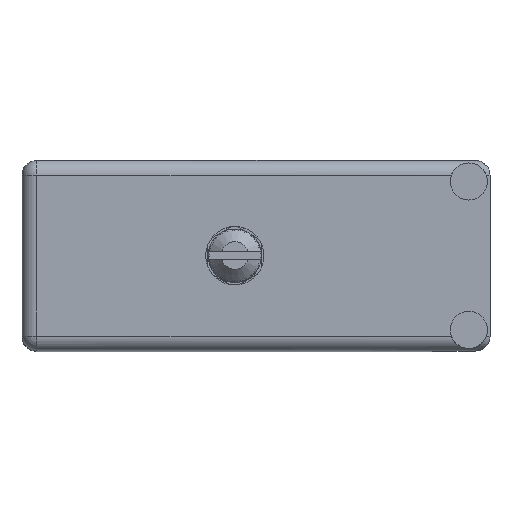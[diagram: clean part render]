
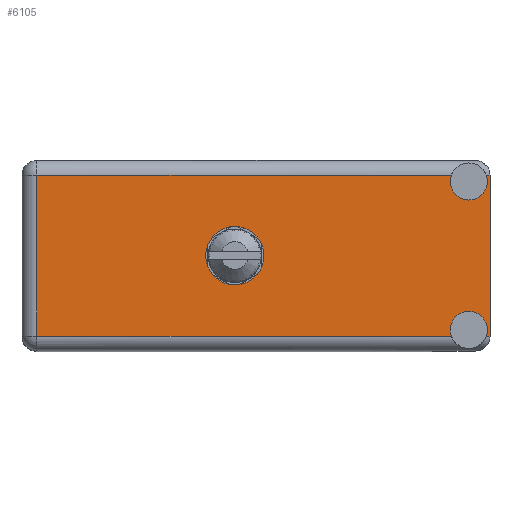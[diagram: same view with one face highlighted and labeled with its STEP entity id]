
A CAD part, top view. The second image highlights one B-rep face of the part: STEP entity #6105.
In plain terms, the highlighted face is planar.
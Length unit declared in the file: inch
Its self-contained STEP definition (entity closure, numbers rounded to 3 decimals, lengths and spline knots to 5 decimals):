
#167 = EDGE_CURVE ( 'NONE', #18167, #98111, #81407, .T. ) ;
#2049 = ORIENTED_EDGE ( 'NONE', *, *, #29045, .T. ) ;
#2720 = CIRCLE ( 'NONE', #59453, 0.0875 ) ;
#3264 = DIRECTION ( 'NONE',  ( 0., 0., 1. ) ) ;
#5481 = CARTESIAN_POINT ( 'NONE',  ( 2.108, 1.566, -0.0995 ) ) ;
#6029 = DIRECTION ( 'NONE',  ( 1., 0., 0. ) ) ;
#6105 = ADVANCED_FACE ( 'NONE', ( #53338, #6647 ), #45706, .T. ) ;
#6292 = VECTOR ( 'NONE', #83411, 39.37008 ) ;
#6294 = AXIS2_PLACEMENT_3D ( 'NONE', #74366, #57599, #89124 ) ;
#6647 = FACE_OUTER_BOUND ( 'NONE', #37424, .T. ) ;
#7308 = DIRECTION ( 'NONE',  ( 0., 0., 1. ) ) ;
#8499 = VERTEX_POINT ( 'NONE', #96741 ) ;
#9598 = ORIENTED_EDGE ( 'NONE', *, *, #73943, .T. ) ;
#11935 = ORIENTED_EDGE ( 'NONE', *, *, #15092, .F. ) ;
#12194 = VERTEX_POINT ( 'NONE', #40960 ) ;
#14160 = VECTOR ( 'NONE', #81929, 39.37008 ) ;
#14945 = ORIENTED_EDGE ( 'NONE', *, *, #33835, .F. ) ;
#15092 = EDGE_CURVE ( 'NONE', #77803, #8499, #61618, .T. ) ;
#16746 = CARTESIAN_POINT ( 'NONE',  ( 2.02562, 1.566, -0.07 ) ) ;
#18047 = EDGE_CURVE ( 'NONE', #32101, #18167, #29146, .T. ) ;
#18167 = VERTEX_POINT ( 'NONE', #63089 ) ;
#18726 = DIRECTION ( 'NONE',  ( 0., 1., 0. ) ) ;
#19003 = DIRECTION ( 'NONE',  ( 0., 1., 0. ) ) ;
#19771 = CARTESIAN_POINT ( 'NONE',  ( 2.108, 1.566, -0.0995 ) ) ;
#21005 = CARTESIAN_POINT ( 'NONE',  ( 1.004, 1.566, -0.312 ) ) ;
#23653 = AXIS2_PLACEMENT_3D ( 'NONE', #79051, #95802, #87690 ) ;
#26522 = VECTOR ( 'NONE', #88206, 39.37008 ) ;
#28844 = VERTEX_POINT ( 'NONE', #21005 ) ;
#28890 = CIRCLE ( 'NONE', #41594, 0.1375 ) ;
#29045 = EDGE_CURVE ( 'NONE', #98111, #50592, #42604, .T. ) ;
#29146 = LINE ( 'NONE', #60066, #6292 ) ;
#29497 = DIRECTION ( 'NONE',  ( 0., 0., 1. ) ) ;
#29644 = CARTESIAN_POINT ( 'NONE',  ( 0.07, 1.566, -0.07 ) ) ;
#32101 = VERTEX_POINT ( 'NONE', #44462 ) ;
#32908 = ORIENTED_EDGE ( 'NONE', *, *, #60147, .T. ) ;
#33835 = EDGE_CURVE ( 'NONE', #32101, #92286, #97107, .T. ) ;
#33897 = CARTESIAN_POINT ( 'NONE',  ( 0., 1.566, -0.829 ) ) ;
#36621 = VECTOR ( 'NONE', #6029, 39.37008 ) ;
#37424 = EDGE_LOOP ( 'NONE', ( #2049, #88988, #90297, #32908, #11935, #9598, #80236, #14945, #94966, #97171 ) ) ;
#37612 = DIRECTION ( 'NONE',  ( 0., 1., 0. ) ) ;
#40960 = CARTESIAN_POINT ( 'NONE',  ( 2.19038, 1.566, -0.829 ) ) ;
#41594 = AXIS2_PLACEMENT_3D ( 'NONE', #70141, #61550, #92561 ) ;
#41675 = AXIS2_PLACEMENT_3D ( 'NONE', #90568, #19003, #3264 ) ;
#42604 = LINE ( 'NONE', #90348, #84325 ) ;
#44462 = CARTESIAN_POINT ( 'NONE',  ( 2.02562, 1.566, -0.829 ) ) ;
#45706 = PLANE ( 'NONE',  #98157 ) ;
#46573 = EDGE_CURVE ( 'NONE', #28844, #48893, #83858, .T. ) ;
#48128 = EDGE_CURVE ( 'NONE', #48893, #28844, #28890, .T. ) ;
#48893 = VERTEX_POINT ( 'NONE', #71758 ) ;
#48980 = ORIENTED_EDGE ( 'NONE', *, *, #46573, .F. ) ;
#49653 = DIRECTION ( 'NONE',  ( 0., 0., 1. ) ) ;
#50592 = VERTEX_POINT ( 'NONE', #16746 ) ;
#51192 = DIRECTION ( 'NONE',  ( 0., 1., 0. ) ) ;
#52324 = CARTESIAN_POINT ( 'NONE',  ( 2.108, 1.566, -0.187 ) ) ;
#52597 = VERTEX_POINT ( 'NONE', #52324 ) ;
#53338 = FACE_BOUND ( 'NONE', #90382, .T. ) ;
#53491 = CARTESIAN_POINT ( 'NONE',  ( 2.208, 1.566, 0. ) ) ;
#57599 = DIRECTION ( 'NONE',  ( 0., 1., 0. ) ) ;
#58346 = DIRECTION ( 'NONE',  ( 1., 0., 0. ) ) ;
#59453 = AXIS2_PLACEMENT_3D ( 'NONE', #19771, #51192, #66448 ) ;
#60066 = CARTESIAN_POINT ( 'NONE',  ( 0., 1.566, -0.829 ) ) ;
#60147 = EDGE_CURVE ( 'NONE', #83844, #8499, #83677, .T. ) ;
#60887 = VECTOR ( 'NONE', #7308, 39.37008 ) ;
#61550 = DIRECTION ( 'NONE',  ( 0., 1., 0. ) ) ;
#61618 = LINE ( 'NONE', #53491, #60887 ) ;
#63089 = CARTESIAN_POINT ( 'NONE',  ( 0.07, 1.566, -0.829 ) ) ;
#64164 = EDGE_CURVE ( 'NONE', #52597, #50592, #96614, .T. ) ;
#64333 = LINE ( 'NONE', #33897, #26522 ) ;
#65685 = CARTESIAN_POINT ( 'NONE',  ( 0.07, 1.566, -0.899 ) ) ;
#65789 = AXIS2_PLACEMENT_3D ( 'NONE', #5481, #18726, #49653 ) ;
#66448 = DIRECTION ( 'NONE',  ( 0., 0., 1. ) ) ;
#69837 = EDGE_CURVE ( 'NONE', #92286, #12194, #88396, .T. ) ;
#70141 = CARTESIAN_POINT ( 'NONE',  ( 1.004, 1.566, -0.4495 ) ) ;
#71758 = CARTESIAN_POINT ( 'NONE',  ( 1.004, 1.566, -0.587 ) ) ;
#73943 = EDGE_CURVE ( 'NONE', #77803, #12194, #64333, .T. ) ;
#74366 = CARTESIAN_POINT ( 'NONE',  ( 2.108, 1.566, -0.7995 ) ) ;
#74615 = CARTESIAN_POINT ( 'NONE',  ( 2.19038, 1.566, -0.07 ) ) ;
#75050 = CARTESIAN_POINT ( 'NONE',  ( 2.208, 1.566, -0.07 ) ) ;
#76131 = EDGE_CURVE ( 'NONE', #83844, #52597, #2720, .T. ) ;
#77803 = VERTEX_POINT ( 'NONE', #98402 ) ;
#79051 = CARTESIAN_POINT ( 'NONE',  ( 2.108, 1.566, -0.7995 ) ) ;
#80236 = ORIENTED_EDGE ( 'NONE', *, *, #69837, .F. ) ;
#81407 = LINE ( 'NONE', #65685, #14160 ) ;
#81929 = DIRECTION ( 'NONE',  ( 0., 0., 1. ) ) ;
#82298 = CARTESIAN_POINT ( 'NONE',  ( 0., 1.566, -0.899 ) ) ;
#83411 = DIRECTION ( 'NONE',  ( -1., 0., 0. ) ) ;
#83677 = LINE ( 'NONE', #75050, #36621 ) ;
#83844 = VERTEX_POINT ( 'NONE', #74615 ) ;
#83858 = CIRCLE ( 'NONE', #41675, 0.1375 ) ;
#84325 = VECTOR ( 'NONE', #58346, 39.37008 ) ;
#85329 = CARTESIAN_POINT ( 'NONE',  ( 2.108, 1.566, -0.712 ) ) ;
#87690 = DIRECTION ( 'NONE',  ( 0., 0., 1. ) ) ;
#88206 = DIRECTION ( 'NONE',  ( -1., 0., 0. ) ) ;
#88396 = CIRCLE ( 'NONE', #23653, 0.0875 ) ;
#88988 = ORIENTED_EDGE ( 'NONE', *, *, #64164, .F. ) ;
#89124 = DIRECTION ( 'NONE',  ( 0., 0., 1. ) ) ;
#90297 = ORIENTED_EDGE ( 'NONE', *, *, #76131, .F. ) ;
#90348 = CARTESIAN_POINT ( 'NONE',  ( 2.208, 1.566, -0.07 ) ) ;
#90382 = EDGE_LOOP ( 'NONE', ( #48980, #94595 ) ) ;
#90568 = CARTESIAN_POINT ( 'NONE',  ( 1.004, 1.566, -0.4495 ) ) ;
#92286 = VERTEX_POINT ( 'NONE', #85329 ) ;
#92561 = DIRECTION ( 'NONE',  ( 0., 0., 1. ) ) ;
#94595 = ORIENTED_EDGE ( 'NONE', *, *, #48128, .F. ) ;
#94966 = ORIENTED_EDGE ( 'NONE', *, *, #18047, .T. ) ;
#95802 = DIRECTION ( 'NONE',  ( 0., 1., 0. ) ) ;
#96614 = CIRCLE ( 'NONE', #65789, 0.0875 ) ;
#96741 = CARTESIAN_POINT ( 'NONE',  ( 2.208, 1.566, -0.07 ) ) ;
#97107 = CIRCLE ( 'NONE', #6294, 0.0875 ) ;
#97171 = ORIENTED_EDGE ( 'NONE', *, *, #167, .T. ) ;
#98111 = VERTEX_POINT ( 'NONE', #29644 ) ;
#98157 = AXIS2_PLACEMENT_3D ( 'NONE', #82298, #37612, #29497 ) ;
#98402 = CARTESIAN_POINT ( 'NONE',  ( 2.208, 1.566, -0.829 ) ) ;
